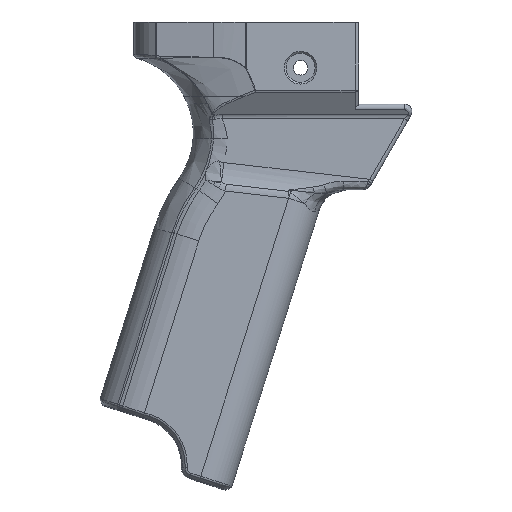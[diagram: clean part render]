
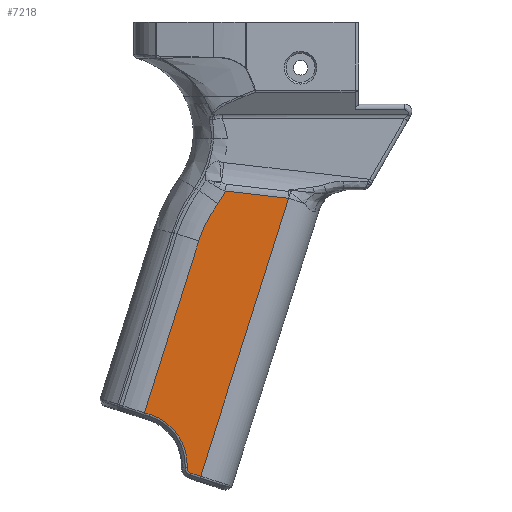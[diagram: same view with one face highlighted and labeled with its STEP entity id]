
A CAD part, front view. The second image highlights one B-rep face of the part: STEP entity #7218.
In plain terms, the highlighted planar face has unit normal (0, -1, 0).
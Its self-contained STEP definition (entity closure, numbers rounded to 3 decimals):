
#214=B_SPLINE_CURVE_WITH_KNOTS('',3,(#15004,#15005,#15006,#15007),
 .UNSPECIFIED.,.F.,.F.,(4,4),(-0.018,0.),
 .UNSPECIFIED.);
#375=PLANE('',#7896);
#661=LINE('',#14348,#1052);
#663=LINE('',#14366,#1054);
#671=LINE('',#14680,#1062);
#704=LINE('',#15009,#1095);
#705=LINE('',#15014,#1096);
#1052=VECTOR('',#9030,10.);
#1054=VECTOR('',#9052,10.);
#1062=VECTOR('',#9080,10.);
#1095=VECTOR('',#9293,10.);
#1096=VECTOR('',#9298,10.);
#1642=FACE_OUTER_BOUND('',#2114,.T.);
#2114=EDGE_LOOP('',(#5640,#5641,#5642,#5643,#5644,#5645,#5646,#5647,#5648,
#5649));
#2591=CIRCLE('',#7790,1.419);
#2594=CIRCLE('',#7794,14.581);
#2648=CIRCLE('',#7897,34.246);
#2649=CIRCLE('',#7898,37.23);
#3114=VERTEX_POINT('',#14328);
#3116=VERTEX_POINT('',#14344);
#3118=VERTEX_POINT('',#14350);
#3120=VERTEX_POINT('',#14356);
#3122=VERTEX_POINT('',#14362);
#3140=VERTEX_POINT('',#14675);
#3179=VERTEX_POINT('',#15003);
#3180=VERTEX_POINT('',#15008);
#3181=VERTEX_POINT('',#15010);
#3182=VERTEX_POINT('',#15012);
#3938=EDGE_CURVE('',#3114,#3116,#661,.T.);
#3941=EDGE_CURVE('',#3116,#3118,#2591,.T.);
#3944=EDGE_CURVE('',#3118,#3120,#2594,.T.);
#3947=EDGE_CURVE('',#3120,#3122,#663,.T.);
#3976=EDGE_CURVE('',#3140,#3114,#671,.T.);
#4062=EDGE_CURVE('',#3179,#3140,#214,.T.);
#4063=EDGE_CURVE('',#3180,#3179,#704,.T.);
#4064=EDGE_CURVE('',#3181,#3180,#2648,.T.);
#4065=EDGE_CURVE('',#3182,#3181,#2649,.T.);
#4066=EDGE_CURVE('',#3122,#3182,#705,.T.);
#5640=ORIENTED_EDGE('',*,*,#3938,.F.);
#5641=ORIENTED_EDGE('',*,*,#3976,.F.);
#5642=ORIENTED_EDGE('',*,*,#4062,.F.);
#5643=ORIENTED_EDGE('',*,*,#4063,.F.);
#5644=ORIENTED_EDGE('',*,*,#4064,.F.);
#5645=ORIENTED_EDGE('',*,*,#4065,.F.);
#5646=ORIENTED_EDGE('',*,*,#4066,.F.);
#5647=ORIENTED_EDGE('',*,*,#3947,.F.);
#5648=ORIENTED_EDGE('',*,*,#3944,.F.);
#5649=ORIENTED_EDGE('',*,*,#3941,.F.);
#7218=ADVANCED_FACE('',(#1642),#375,.T.);
#7790=AXIS2_PLACEMENT_3D('',#14354,#9037,#9038);
#7794=AXIS2_PLACEMENT_3D('',#14360,#9045,#9046);
#7896=AXIS2_PLACEMENT_3D('',#15002,#9291,#9292);
#7897=AXIS2_PLACEMENT_3D('',#15011,#9294,#9295);
#7898=AXIS2_PLACEMENT_3D('',#15013,#9296,#9297);
#9030=DIRECTION('',(-0.953,0.,0.301));
#9037=DIRECTION('center_axis',(0.,1.,0.));
#9038=DIRECTION('ref_axis',(-0.822,0.,-0.569));
#9045=DIRECTION('center_axis',(0.,-1.,0.));
#9046=DIRECTION('ref_axis',(0.822,0.,0.569));
#9052=DIRECTION('',(-0.953,0.,0.301));
#9080=DIRECTION('',(-0.301,0.,-0.953));
#9291=DIRECTION('center_axis',(0.,-1.,0.));
#9292=DIRECTION('ref_axis',(1.,0.,0.));
#9293=DIRECTION('',(0.993,0.,-0.114));
#9294=DIRECTION('center_axis',(0.,-1.,0.));
#9295=DIRECTION('ref_axis',(0.833,0.,-0.553));
#9296=DIRECTION('center_axis',(0.,1.,0.));
#9297=DIRECTION('ref_axis',(-0.888,0.,0.459));
#9298=DIRECTION('',(0.301,0.,0.953));
#14328=CARTESIAN_POINT('',(-178.613,3.068,-127.473));
#14344=CARTESIAN_POINT('',(-181.352,3.068,-126.607));
#14348=CARTESIAN_POINT('',(-176.104,3.068,-128.266));
#14350=CARTESIAN_POINT('',(-182.341,3.068,-125.178));
#14354=CARTESIAN_POINT('Origin',(-180.924,3.068,-125.254));
#14356=CARTESIAN_POINT('',(-192.507,3.068,-110.496));
#14360=CARTESIAN_POINT('Origin',(-196.901,3.068,-124.399));
#14362=CARTESIAN_POINT('',(-194.075,3.068,-110.));
#14366=CARTESIAN_POINT('',(-174.614,3.068,-116.151));
#14675=CARTESIAN_POINT('',(-154.447,3.068,-51.022));
#14680=CARTESIAN_POINT('',(-158.165,3.068,-62.785));
#15002=CARTESIAN_POINT('Origin',(-159.401,3.068,-74.198));
#15003=CARTESIAN_POINT('',(-154.624,3.068,-50.984));
#15004=CARTESIAN_POINT('Ctrl Pts',(-154.624,3.068,-50.984));
#15005=CARTESIAN_POINT('Ctrl Pts',(-154.564,3.068,-50.991));
#15006=CARTESIAN_POINT('Ctrl Pts',(-154.505,3.068,-51.003));
#15007=CARTESIAN_POINT('Ctrl Pts',(-154.447,3.068,-51.022));
#15008=CARTESIAN_POINT('',(-171.8,3.068,-49.012));
#15009=CARTESIAN_POINT('',(-144.123,3.068,-52.19));
#15010=CARTESIAN_POINT('',(-173.881,3.068,-52.467));
#15011=CARTESIAN_POINT('Origin',(-202.126,3.068,-33.103));
#15012=CARTESIAN_POINT('',(-179.14,3.068,-62.751));
#15013=CARTESIAN_POINT('Origin',(-143.765,3.068,-74.355));
#15014=CARTESIAN_POINT('',(-179.058,3.068,-62.491));
